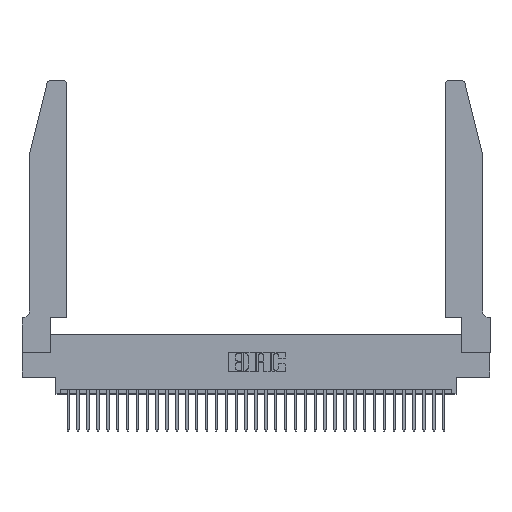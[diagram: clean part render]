
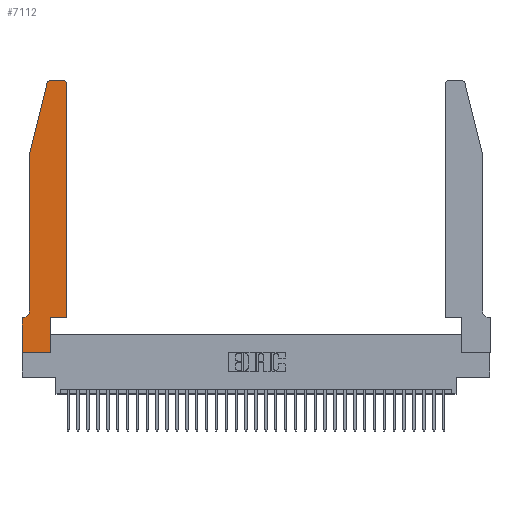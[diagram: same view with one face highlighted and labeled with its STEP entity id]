
A CAD part, top view. The second image highlights one B-rep face of the part: STEP entity #7112.
In plain terms, the highlighted planar face has unit normal (0, 0, 1).
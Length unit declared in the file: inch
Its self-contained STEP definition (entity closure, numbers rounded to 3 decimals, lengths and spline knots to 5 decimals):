
#522 = VECTOR ( 'NONE', #9378, 39.37008 ) ;
#647 = CARTESIAN_POINT ( 'NONE',  ( 0.4505, 0.35, 0.37 ) ) ;
#999 = CIRCLE ( 'NONE', #4162, 0.03 ) ;
#2772 = CARTESIAN_POINT ( 'NONE',  ( 0.0755, 2., 0.37 ) ) ;
#3407 = CARTESIAN_POINT ( 'NONE',  ( 0.4205, 2.75, 0.37 ) ) ;
#3428 = VERTEX_POINT ( 'NONE', #33272 ) ;
#3725 = ORIENTED_EDGE ( 'NONE', *, *, #6539, .T. ) ;
#4105 = CARTESIAN_POINT ( 'NONE',  ( 0.284, 2.72, 0.37 ) ) ;
#4162 = AXIS2_PLACEMENT_3D ( 'NONE', #4105, #23481, #6941 ) ;
#4727 = EDGE_CURVE ( 'NONE', #23499, #6794, #32984, .T. ) ;
#4878 = PLANE ( 'NONE',  #25303 ) ;
#5065 = DIRECTION ( 'NONE',  ( -1., 0., 0. ) ) ;
#5636 = DIRECTION ( 'NONE',  ( 0., -1., 0. ) ) ;
#5698 = CIRCLE ( 'NONE', #26613, 0.07 ) ;
#6512 = CARTESIAN_POINT ( 'NONE',  ( 0.2865, 0.35, 0.37 ) ) ;
#6539 = EDGE_CURVE ( 'NONE', #34281, #27936, #29848, .T. ) ;
#6562 = CARTESIAN_POINT ( 'NONE',  ( 0.0755, 0.35, 0.37 ) ) ;
#6794 = VERTEX_POINT ( 'NONE', #3407 ) ;
#6941 = DIRECTION ( 'NONE',  ( 1., 0., 0. ) ) ;
#6958 = VECTOR ( 'NONE', #35885, 39.37008 ) ;
#7112 = ADVANCED_FACE ( 'NONE', ( #16947 ), #4878, .T. ) ;
#7145 = LINE ( 'NONE', #2772, #20138 ) ;
#7712 = DIRECTION ( 'NONE',  ( 0., 0., 1. ) ) ;
#8124 = CARTESIAN_POINT ( 'NONE',  ( 0.4505, 0.35, 0.37 ) ) ;
#8410 = CARTESIAN_POINT ( 'NONE',  ( 0., 0., 0.37 ) ) ;
#8841 = ORIENTED_EDGE ( 'NONE', *, *, #14017, .T. ) ;
#9378 = DIRECTION ( 'NONE',  ( -1., 0., 0. ) ) ;
#10157 = DIRECTION ( 'NONE',  ( 0., 0., 1. ) ) ;
#10833 = CARTESIAN_POINT ( 'NONE',  ( 0.4505, 0.35, 0.37 ) ) ;
#11044 = ORIENTED_EDGE ( 'NONE', *, *, #19884, .T. ) ;
#11814 = CARTESIAN_POINT ( 'NONE',  ( 0.284, 2.75, 0.37 ) ) ;
#13425 = CARTESIAN_POINT ( 'NONE',  ( 0.0055, 0.42, 0.37 ) ) ;
#13571 = CARTESIAN_POINT ( 'NONE',  ( 0.0755, 2., 0.37 ) ) ;
#14017 = EDGE_CURVE ( 'NONE', #28565, #31364, #32619, .T. ) ;
#14075 = EDGE_CURVE ( 'NONE', #3428, #25066, #15371, .T. ) ;
#14097 = VECTOR ( 'NONE', #20125, 39.37008 ) ;
#14557 = CARTESIAN_POINT ( 'NONE',  ( 0.2865, 0., 0.37 ) ) ;
#14801 = EDGE_LOOP ( 'NONE', ( #11044, #30427, #3725, #22124, #20249, #19584, #33185, #25189, #31744, #8841, #21456, #27510 ) ) ;
#15371 = LINE ( 'NONE', #6562, #522 ) ;
#15987 = DIRECTION ( 'NONE',  ( 1., 0., 0. ) ) ;
#16107 = CARTESIAN_POINT ( 'NONE',  ( 0.2605, 2.75, 0.37 ) ) ;
#16185 = DIRECTION ( 'NONE',  ( -1., 0., 0. ) ) ;
#16327 = DIRECTION ( 'NONE',  ( -0.239, -0.971, 0. ) ) ;
#16432 = EDGE_CURVE ( 'NONE', #25066, #29476, #20822, .T. ) ;
#16947 = FACE_OUTER_BOUND ( 'NONE', #14801, .T. ) ;
#17871 = EDGE_CURVE ( 'NONE', #32397, #28565, #32773, .T. ) ;
#19584 = ORIENTED_EDGE ( 'NONE', *, *, #14075, .T. ) ;
#19884 = EDGE_CURVE ( 'NONE', #6794, #28438, #27378, .T. ) ;
#20125 = DIRECTION ( 'NONE',  ( 1., 0., 0. ) ) ;
#20138 = VECTOR ( 'NONE', #5636, 39.37008 ) ;
#20238 = VECTOR ( 'NONE', #30208, 39.37008 ) ;
#20249 = ORIENTED_EDGE ( 'NONE', *, *, #30658, .T. ) ;
#20822 = LINE ( 'NONE', #32986, #6958 ) ;
#21120 = LINE ( 'NONE', #8124, #20238 ) ;
#21456 = ORIENTED_EDGE ( 'NONE', *, *, #24388, .T. ) ;
#21501 = CARTESIAN_POINT ( 'NONE',  ( 0., 0.35, 0.37 ) ) ;
#21772 = CARTESIAN_POINT ( 'NONE',  ( 0., 0., 0.37 ) ) ;
#21971 = VECTOR ( 'NONE', #15987, 39.37008 ) ;
#22088 = CARTESIAN_POINT ( 'NONE',  ( 0.0755, 0.42, 0.37 ) ) ;
#22124 = ORIENTED_EDGE ( 'NONE', *, *, #25792, .T. ) ;
#23073 = DIRECTION ( 'NONE',  ( 0., 1., 0. ) ) ;
#23350 = CARTESIAN_POINT ( 'NONE',  ( 0.2865, 0.35, 0.37 ) ) ;
#23377 = CARTESIAN_POINT ( 'NONE',  ( 0.4505, 2.72, 0.37 ) ) ;
#23481 = DIRECTION ( 'NONE',  ( 0., 0., 1. ) ) ;
#23499 = VERTEX_POINT ( 'NONE', #23377 ) ;
#24375 = EDGE_CURVE ( 'NONE', #29476, #32397, #29305, .T. ) ;
#24388 = EDGE_CURVE ( 'NONE', #31364, #23499, #21120, .T. ) ;
#25066 = VERTEX_POINT ( 'NONE', #35591 ) ;
#25189 = ORIENTED_EDGE ( 'NONE', *, *, #24375, .T. ) ;
#25303 = AXIS2_PLACEMENT_3D ( 'NONE', #21501, #7712, #27001 ) ;
#25431 = VECTOR ( 'NONE', #23073, 39.37008 ) ;
#25471 = EDGE_CURVE ( 'NONE', #28438, #34281, #999, .T. ) ;
#25792 = EDGE_CURVE ( 'NONE', #27936, #30729, #7145, .T. ) ;
#26398 = CARTESIAN_POINT ( 'NONE',  ( 0.0755, 2., 0.37 ) ) ;
#26613 = AXIS2_PLACEMENT_3D ( 'NONE', #13425, #32692, #16185 ) ;
#26646 = CARTESIAN_POINT ( 'NONE',  ( 0.4205, 2.72, 0.37 ) ) ;
#27001 = DIRECTION ( 'NONE',  ( 1., 0., 0. ) ) ;
#27378 = LINE ( 'NONE', #16107, #34770 ) ;
#27510 = ORIENTED_EDGE ( 'NONE', *, *, #4727, .T. ) ;
#27936 = VERTEX_POINT ( 'NONE', #26398 ) ;
#28281 = AXIS2_PLACEMENT_3D ( 'NONE', #26646, #10157, #29445 ) ;
#28438 = VERTEX_POINT ( 'NONE', #11814 ) ;
#28565 = VERTEX_POINT ( 'NONE', #23350 ) ;
#29305 = LINE ( 'NONE', #21772, #21971 ) ;
#29445 = DIRECTION ( 'NONE',  ( 1., 0., 0. ) ) ;
#29476 = VERTEX_POINT ( 'NONE', #8410 ) ;
#29848 = LINE ( 'NONE', #13571, #34595 ) ;
#30208 = DIRECTION ( 'NONE',  ( 0., 1., 0. ) ) ;
#30427 = ORIENTED_EDGE ( 'NONE', *, *, #25471, .T. ) ;
#30658 = EDGE_CURVE ( 'NONE', #30729, #3428, #5698, .T. ) ;
#30729 = VERTEX_POINT ( 'NONE', #22088 ) ;
#31364 = VERTEX_POINT ( 'NONE', #10833 ) ;
#31744 = ORIENTED_EDGE ( 'NONE', *, *, #17871, .T. ) ;
#32397 = VERTEX_POINT ( 'NONE', #14557 ) ;
#32619 = LINE ( 'NONE', #647, #14097 ) ;
#32692 = DIRECTION ( 'NONE',  ( 0., 0., -1. ) ) ;
#32773 = LINE ( 'NONE', #6512, #25431 ) ;
#32984 = CIRCLE ( 'NONE', #28281, 0.03 ) ;
#32986 = CARTESIAN_POINT ( 'NONE',  ( 0., 0., 0.37 ) ) ;
#33185 = ORIENTED_EDGE ( 'NONE', *, *, #16432, .T. ) ;
#33272 = CARTESIAN_POINT ( 'NONE',  ( 0.0055, 0.35, 0.37 ) ) ;
#33956 = CARTESIAN_POINT ( 'NONE',  ( 0.25487, 2.72718, 0.37 ) ) ;
#34281 = VERTEX_POINT ( 'NONE', #33956 ) ;
#34595 = VECTOR ( 'NONE', #16327, 39.37008 ) ;
#34770 = VECTOR ( 'NONE', #5065, 39.37008 ) ;
#35591 = CARTESIAN_POINT ( 'NONE',  ( 0., 0.35, 0.37 ) ) ;
#35885 = DIRECTION ( 'NONE',  ( 0., -1., 0. ) ) ;
